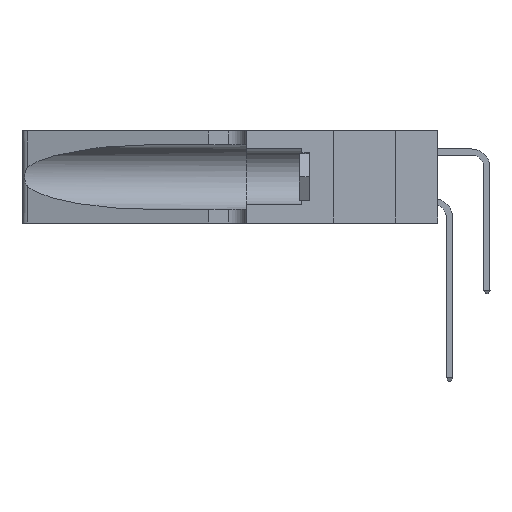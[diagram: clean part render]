
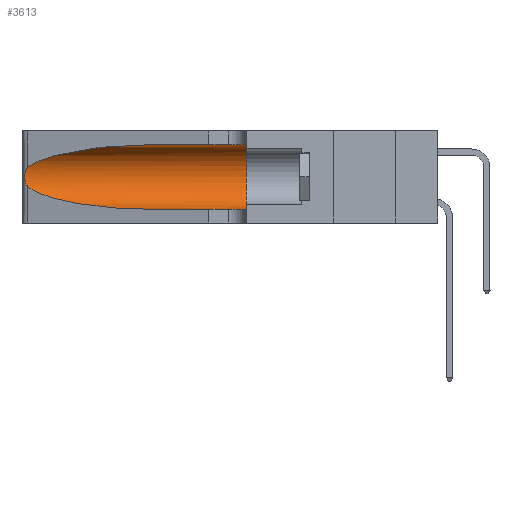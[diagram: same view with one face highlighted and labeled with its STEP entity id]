
A CAD part, left-side view. The second image highlights one B-rep face of the part: STEP entity #3613.
In plain terms, the highlighted cylindrical face has radius 3.308 mm (diameter 6.617 mm), a partial arc.
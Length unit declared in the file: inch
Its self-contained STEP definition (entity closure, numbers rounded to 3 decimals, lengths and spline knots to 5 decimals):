
#65 = CARTESIAN_POINT ( 'NONE',  ( 0.25487, 1.22718, 0.22369 ) ) ;
#146 = CARTESIAN_POINT ( 'NONE',  ( 0.18966, 0.96281, 0.31525 ) ) ;
#373 = CARTESIAN_POINT ( 'NONE',  ( 0.1305, 0.72297, 0.31525 ) ) ;
#775 = ORIENTED_EDGE ( 'NONE', *, *, #16122, .T. ) ;
#791 = CARTESIAN_POINT ( 'NONE',  ( 0.25555, 1.22993, 0.14849 ) ) ;
#820 = VECTOR ( 'NONE', #15936, 39.37008 ) ;
#1121 = CARTESIAN_POINT ( 'NONE',  ( 0.25789, 1.23486, 0.15765 ) ) ;
#1589 = ORIENTED_EDGE ( 'NONE', *, *, #15337, .T. ) ;
#2662 = CARTESIAN_POINT ( 'NONE',  ( 0.25487, 1.22718, 0.14631 ) ) ;
#2690 = LINE ( 'NONE', #10297, #16241 ) ;
#2914 = CARTESIAN_POINT ( 'NONE',  ( 0.25487, 1.22718, 0.22369 ) ) ;
#3171 =( BOUNDED_CURVE ( )  B_SPLINE_CURVE ( 3, ( #373, #146, #11336, #65 ),
 .UNSPECIFIED., .F., .F. ) 
 B_SPLINE_CURVE_WITH_KNOTS ( ( 4, 4 ),
 ( 1.5708, 2.84003 ),
 .UNSPECIFIED. ) 
 CURVE ( )  GEOMETRIC_REPRESENTATION_ITEM ( )  RATIONAL_B_SPLINE_CURVE ( ( 1., 0.87, 0.87, 1. ) ) 
 REPRESENTATION_ITEM ( '' )  );
#3598 = ORIENTED_EDGE ( 'NONE', *, *, #4137, .F. ) ;
#3613 = ADVANCED_FACE ( 'NONE', ( #14483 ), #13298, .F. ) ;
#4137 = EDGE_CURVE ( 'NONE', #22814, #10068, #2690, .T. ) ;
#4763 = CARTESIAN_POINT ( 'NONE',  ( 0.26018, 1.23835, 0.19895 ) ) ;
#5152 = EDGE_LOOP ( 'NONE', ( #1589, #10346, #775, #16917, #7745, #3598 ) ) ;
#5635 = CARTESIAN_POINT ( 'NONE',  ( 0.25487, 1.22718, 0.14631 ) ) ;
#5681 =( BOUNDED_CURVE ( )  B_SPLINE_CURVE ( 3, ( #11655, #9996, #10162, #23076 ),
 .UNSPECIFIED., .F., .F. ) 
 B_SPLINE_CURVE_WITH_KNOTS ( ( 4, 4 ),
 ( 3.44316, 4.71239 ),
 .UNSPECIFIED. ) 
 CURVE ( )  GEOMETRIC_REPRESENTATION_ITEM ( )  RATIONAL_B_SPLINE_CURVE ( ( 1., 0.87, 0.87, 1. ) ) 
 REPRESENTATION_ITEM ( '' )  );
#6397 = CARTESIAN_POINT ( 'NONE',  ( 0.25555, 1.22994, 0.2215 ) ) ;
#7055 = CARTESIAN_POINT ( 'NONE',  ( 0.1305, 1.61858, 0.05475 ) ) ;
#7745 = ORIENTED_EDGE ( 'NONE', *, *, #19232, .F. ) ;
#9382 = DIRECTION ( 'NONE',  ( 0., 0., 1. ) ) ;
#9996 = CARTESIAN_POINT ( 'NONE',  ( 0.2373, 1.15595, 0.08982 ) ) ;
#10007 = CARTESIAN_POINT ( 'NONE',  ( 0.25854, 1.2359, 0.20912 ) ) ;
#10068 = VERTEX_POINT ( 'NONE', #13755 ) ;
#10162 = CARTESIAN_POINT ( 'NONE',  ( 0.18966, 0.96281, 0.05475 ) ) ;
#10297 = CARTESIAN_POINT ( 'NONE',  ( 0.1305, 1.61858, 0.31525 ) ) ;
#10325 = CARTESIAN_POINT ( 'NONE',  ( 0.25856, 1.23593, 0.16098 ) ) ;
#10346 = ORIENTED_EDGE ( 'NONE', *, *, #20531, .T. ) ;
#10599 = CARTESIAN_POINT ( 'NONE',  ( 0.1305, 0.72297, 0.05475 ) ) ;
#11237 = DIRECTION ( 'NONE',  ( 0., 0., -1. ) ) ;
#11336 = CARTESIAN_POINT ( 'NONE',  ( 0.2373, 1.15595, 0.28018 ) ) ;
#11655 = CARTESIAN_POINT ( 'NONE',  ( 0.25487, 1.22718, 0.14631 ) ) ;
#11827 = CARTESIAN_POINT ( 'NONE',  ( 0.25639, 1.23186, 0.15144 ) ) ;
#11997 = AXIS2_PLACEMENT_3D ( 'NONE', #20568, #15085, #9382 ) ;
#12392 = CARTESIAN_POINT ( 'NONE',  ( 0.25487, 1.22718, 0.22369 ) ) ;
#12564 = CIRCLE ( 'NONE', #11997, 0.13025 ) ;
#13087 = VERTEX_POINT ( 'NONE', #10599 ) ;
#13148 = DIRECTION ( 'NONE',  ( 0., -1., 0. ) ) ;
#13298 = CYLINDRICAL_SURFACE ( 'NONE', #13322, 0.13025 ) ;
#13322 = AXIS2_PLACEMENT_3D ( 'NONE', #20508, #13148, #11237 ) ;
#13669 = CARTESIAN_POINT ( 'NONE',  ( 0.25639, 1.23184, 0.21858 ) ) ;
#13755 = CARTESIAN_POINT ( 'NONE',  ( 0.1305, 0.35, 0.31525 ) ) ;
#14483 = FACE_OUTER_BOUND ( 'NONE', #5152, .T. ) ;
#15085 = DIRECTION ( 'NONE',  ( 0., 1., 0. ) ) ;
#15337 = EDGE_CURVE ( 'NONE', #22814, #22679, #3171, .T. ) ;
#15936 = DIRECTION ( 'NONE',  ( 0., -1., 0. ) ) ;
#16006 = VERTEX_POINT ( 'NONE', #19251 ) ;
#16122 = EDGE_CURVE ( 'NONE', #16372, #13087, #5681, .T. ) ;
#16241 = VECTOR ( 'NONE', #19966, 39.37008 ) ;
#16372 = VERTEX_POINT ( 'NONE', #5635 ) ;
#16917 = ORIENTED_EDGE ( 'NONE', *, *, #16970, .T. ) ;
#16970 = EDGE_CURVE ( 'NONE', #13087, #16006, #19008, .T. ) ;
#17621 = CARTESIAN_POINT ( 'NONE',  ( 0.26075, 1.23896, 0.19203 ) ) ;
#17706 = CARTESIAN_POINT ( 'NONE',  ( 0.25787, 1.23484, 0.2124 ) ) ;
#19008 = LINE ( 'NONE', #7055, #820 ) ;
#19232 = EDGE_CURVE ( 'NONE', #10068, #16006, #12564, .T. ) ;
#19251 = CARTESIAN_POINT ( 'NONE',  ( 0.1305, 0.35, 0.05475 ) ) ;
#19966 = DIRECTION ( 'NONE',  ( 0., -1., 0. ) ) ;
#20508 = CARTESIAN_POINT ( 'NONE',  ( 0.1305, 1.61858, 0.185 ) ) ;
#20531 = EDGE_CURVE ( 'NONE', #22679, #16372, #22228, .T. ) ;
#20568 = CARTESIAN_POINT ( 'NONE',  ( 0.1305, 0.35, 0.185 ) ) ;
#21363 = CARTESIAN_POINT ( 'NONE',  ( 0.26017, 1.23833, 0.17102 ) ) ;
#21950 = CARTESIAN_POINT ( 'NONE',  ( 0.1305, 0.72297, 0.31525 ) ) ;
#22228 = B_SPLINE_CURVE_WITH_KNOTS ( 'NONE', 3,
 ( #2914, #6397, #13669, #17706, #10007, #4763, #17621, #22921, #21363, #10325, #1121, #11827, #791, #2662 ),
 .UNSPECIFIED., .F., .F.,
 ( 4, 2, 2, 2, 2, 2, 4 ),
 ( 0., 0.00027, 0.00053, 0.00107, 0.0016, 0.00187, 0.00214 ),
 .UNSPECIFIED. ) ;
#22679 = VERTEX_POINT ( 'NONE', #12392 ) ;
#22814 = VERTEX_POINT ( 'NONE', #21950 ) ;
#22921 = CARTESIAN_POINT ( 'NONE',  ( 0.26075, 1.23896, 0.178 ) ) ;
#23076 = CARTESIAN_POINT ( 'NONE',  ( 0.1305, 0.72297, 0.05475 ) ) ;
